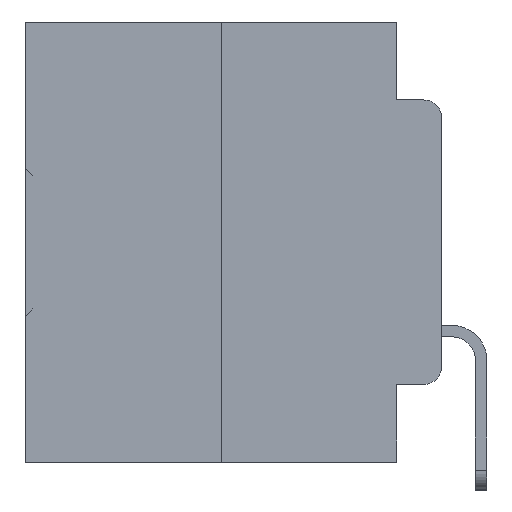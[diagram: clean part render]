
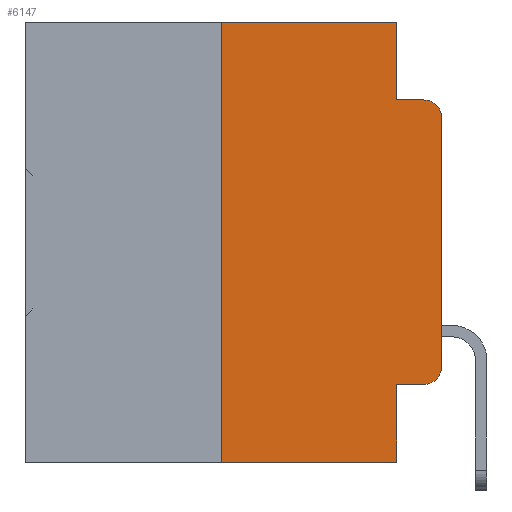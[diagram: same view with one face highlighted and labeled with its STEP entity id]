
A CAD part, left-side view. The second image highlights one B-rep face of the part: STEP entity #6147.
In plain terms, the highlighted planar face has unit normal (-1, 0, 0).
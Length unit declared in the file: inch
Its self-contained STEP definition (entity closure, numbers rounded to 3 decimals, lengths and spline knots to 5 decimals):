
#486 = DIRECTION ( 'NONE',  ( 0., -1., 0. ) ) ;
#1828 = CARTESIAN_POINT ( 'NONE',  ( 0., 0.02, -0.4115 ) ) ;
#1974 = CARTESIAN_POINT ( 'NONE',  ( 0., 0.25, -0.5 ) ) ;
#2962 = CARTESIAN_POINT ( 'NONE',  ( 0., 0., 0. ) ) ;
#3013 = LINE ( 'NONE', #34135, #17139 ) ;
#3827 = CARTESIAN_POINT ( 'NONE',  ( 0., 0.051, 0. ) ) ;
#4892 = CIRCLE ( 'NONE', #30734, 0.02 ) ;
#4923 = VERTEX_POINT ( 'NONE', #26186 ) ;
#5811 = CARTESIAN_POINT ( 'NONE',  ( 0., 0.051, -0.4115 ) ) ;
#5995 = AXIS2_PLACEMENT_3D ( 'NONE', #15078, #23410, #20729 ) ;
#6147 = ADVANCED_FACE ( 'NONE', ( #30505 ), #17892, .F. ) ;
#6259 = ORIENTED_EDGE ( 'NONE', *, *, #7824, .T. ) ;
#6401 = CARTESIAN_POINT ( 'NONE',  ( 0., 0.051, 0. ) ) ;
#6690 = VECTOR ( 'NONE', #23308, 39.37008 ) ;
#6924 = LINE ( 'NONE', #2962, #21067 ) ;
#7143 = VERTEX_POINT ( 'NONE', #5811 ) ;
#7197 = VERTEX_POINT ( 'NONE', #14624 ) ;
#7503 = ORIENTED_EDGE ( 'NONE', *, *, #20489, .T. ) ;
#7518 = VERTEX_POINT ( 'NONE', #1828 ) ;
#7528 = ORIENTED_EDGE ( 'NONE', *, *, #19005, .F. ) ;
#7824 = EDGE_CURVE ( 'NONE', #7518, #4923, #4892, .T. ) ;
#8010 = EDGE_LOOP ( 'NONE', ( #31360, #7503, #26045, #15503, #27342, #34323, #20837, #7528, #29119, #6259 ) ) ;
#8035 = CARTESIAN_POINT ( 'NONE',  ( 0., 0.473, -0.5 ) ) ;
#8360 = CIRCLE ( 'NONE', #33135, 0.02 ) ;
#8952 = DIRECTION ( 'NONE',  ( -1., 0., 0. ) ) ;
#9021 = EDGE_CURVE ( 'NONE', #7143, #7518, #3013, .T. ) ;
#9338 = CARTESIAN_POINT ( 'NONE',  ( 0., 0.02, -0.3915 ) ) ;
#9505 = DIRECTION ( 'NONE',  ( 0., 0., -1. ) ) ;
#11682 = LINE ( 'NONE', #31193, #18303 ) ;
#12042 = VERTEX_POINT ( 'NONE', #30238 ) ;
#12225 = CARTESIAN_POINT ( 'NONE',  ( 0., 0.051, -0.5 ) ) ;
#12228 = DIRECTION ( 'NONE',  ( 0., 0., -1. ) ) ;
#12245 = EDGE_CURVE ( 'NONE', #24452, #29965, #13371, .T. ) ;
#12907 = EDGE_CURVE ( 'NONE', #17321, #25980, #36038, .T. ) ;
#13371 = LINE ( 'NONE', #6401, #6690 ) ;
#13675 = DIRECTION ( 'NONE',  ( 0., -1., 0. ) ) ;
#14624 = CARTESIAN_POINT ( 'NONE',  ( 0., 0., -0.1085 ) ) ;
#15078 = CARTESIAN_POINT ( 'NONE',  ( 0., 0.473, 0. ) ) ;
#15503 = ORIENTED_EDGE ( 'NONE', *, *, #12245, .F. ) ;
#16111 = CARTESIAN_POINT ( 'NONE',  ( 0., 0.051, -0.0885 ) ) ;
#16402 = EDGE_CURVE ( 'NONE', #17321, #20101, #11682, .T. ) ;
#16725 = CARTESIAN_POINT ( 'NONE',  ( 0., 0.473, 0. ) ) ;
#16815 = EDGE_CURVE ( 'NONE', #20101, #24452, #18267, .T. ) ;
#17139 = VECTOR ( 'NONE', #486, 39.37008 ) ;
#17321 = VERTEX_POINT ( 'NONE', #1974 ) ;
#17487 = VECTOR ( 'NONE', #13675, 39.37008 ) ;
#17892 = PLANE ( 'NONE',  #5995 ) ;
#18267 = LINE ( 'NONE', #16725, #33959 ) ;
#18303 = VECTOR ( 'NONE', #34086, 39.37008 ) ;
#19005 = EDGE_CURVE ( 'NONE', #7143, #25980, #22171, .T. ) ;
#20101 = VERTEX_POINT ( 'NONE', #26470 ) ;
#20366 = VECTOR ( 'NONE', #22119, 39.37008 ) ;
#20489 = EDGE_CURVE ( 'NONE', #7197, #12042, #8360, .T. ) ;
#20729 = DIRECTION ( 'NONE',  ( 0., 0., -1. ) ) ;
#20837 = ORIENTED_EDGE ( 'NONE', *, *, #12907, .T. ) ;
#21067 = VECTOR ( 'NONE', #22660, 39.37008 ) ;
#21411 = EDGE_CURVE ( 'NONE', #29965, #12042, #26695, .T. ) ;
#22119 = DIRECTION ( 'NONE',  ( 0., -1., 0. ) ) ;
#22171 = LINE ( 'NONE', #3827, #36108 ) ;
#22660 = DIRECTION ( 'NONE',  ( 0., 0., 1. ) ) ;
#23308 = DIRECTION ( 'NONE',  ( 0., 0., -1. ) ) ;
#23410 = DIRECTION ( 'NONE',  ( 1., 0., 0. ) ) ;
#24452 = VERTEX_POINT ( 'NONE', #27724 ) ;
#24823 = CARTESIAN_POINT ( 'NONE',  ( 0., 0.051, -0.0885 ) ) ;
#25845 = CARTESIAN_POINT ( 'NONE',  ( 0., 0.02, -0.1085 ) ) ;
#25980 = VERTEX_POINT ( 'NONE', #12225 ) ;
#26045 = ORIENTED_EDGE ( 'NONE', *, *, #21411, .F. ) ;
#26186 = CARTESIAN_POINT ( 'NONE',  ( 0., 0., -0.3915 ) ) ;
#26470 = CARTESIAN_POINT ( 'NONE',  ( 0., 0.25, 0. ) ) ;
#26695 = LINE ( 'NONE', #24823, #17487 ) ;
#27269 = EDGE_CURVE ( 'NONE', #4923, #7197, #6924, .T. ) ;
#27342 = ORIENTED_EDGE ( 'NONE', *, *, #16815, .F. ) ;
#27724 = CARTESIAN_POINT ( 'NONE',  ( 0., 0.051, 0. ) ) ;
#28626 = DIRECTION ( 'NONE',  ( 0., 0., -1. ) ) ;
#29010 = DIRECTION ( 'NONE',  ( -1., 0., 0. ) ) ;
#29119 = ORIENTED_EDGE ( 'NONE', *, *, #9021, .T. ) ;
#29965 = VERTEX_POINT ( 'NONE', #16111 ) ;
#30238 = CARTESIAN_POINT ( 'NONE',  ( 0., 0.02, -0.0885 ) ) ;
#30505 = FACE_OUTER_BOUND ( 'NONE', #8010, .T. ) ;
#30734 = AXIS2_PLACEMENT_3D ( 'NONE', #9338, #29010, #12228 ) ;
#31193 = CARTESIAN_POINT ( 'NONE',  ( 0., 0.25, 0. ) ) ;
#31360 = ORIENTED_EDGE ( 'NONE', *, *, #27269, .T. ) ;
#33135 = AXIS2_PLACEMENT_3D ( 'NONE', #25845, #8952, #28626 ) ;
#33959 = VECTOR ( 'NONE', #36251, 39.37008 ) ;
#34086 = DIRECTION ( 'NONE',  ( 0., 0., 1. ) ) ;
#34135 = CARTESIAN_POINT ( 'NONE',  ( 0., 0.051, -0.4115 ) ) ;
#34323 = ORIENTED_EDGE ( 'NONE', *, *, #16402, .F. ) ;
#36038 = LINE ( 'NONE', #8035, #20366 ) ;
#36108 = VECTOR ( 'NONE', #9505, 39.37008 ) ;
#36251 = DIRECTION ( 'NONE',  ( 0., -1., 0. ) ) ;
